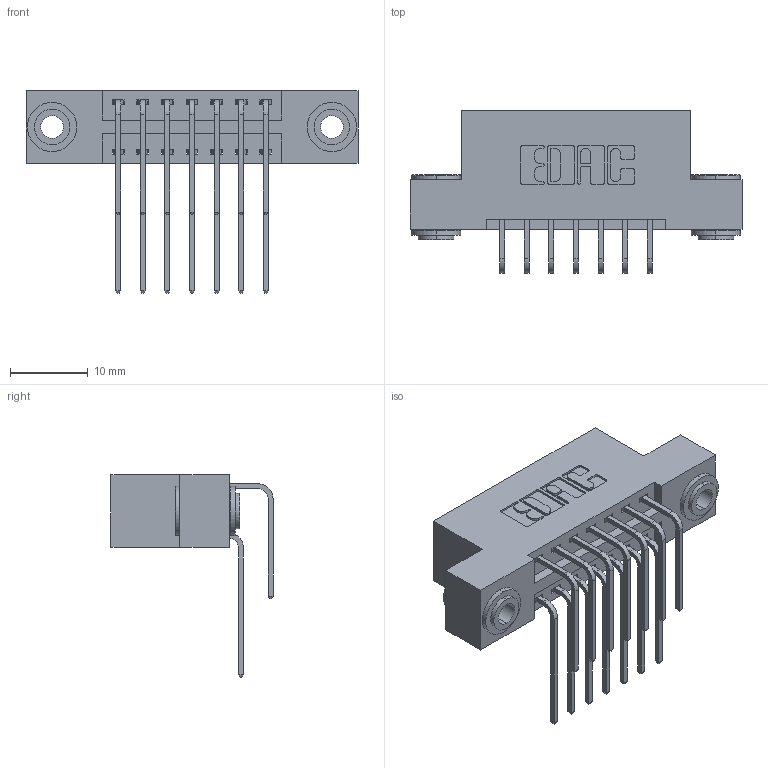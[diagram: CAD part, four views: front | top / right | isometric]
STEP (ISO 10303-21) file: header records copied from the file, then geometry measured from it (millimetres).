
FILE_DESCRIPTION (( 'STEP AP203' ), '1' );
FILE_NAME ('396-014-559-203.STEP', '2018-08-31T11:12:21', ( '' ), ( '' ), 'SwSTEP 2.0', 'SolidWorks 2016', '' );
FILE_SCHEMA (( 'CONFIG_CONTROL_DESIGN' ));
Length unit declared in the file: inch
Products named in the file (5): 346 Part_Flush Mounting Lugs - 0.156 Dia-TH; 345-292-001_558 559 Tail - 1; 345-292-001_559 Tail - 2; 345-250-002_345-250-002-102; 396-014-559-203
Assembly tree (17 placements, depth 2):
  396-014-559-203
    346 Part_Flush Mounting Lugs - 0.156 Dia-TH
    345-292-001_558 559 Tail - 1  x7
    345-292-001_559 Tail - 2  x7
    345-250-002_345-250-002-102  x2
Bounding box: 42.8 x 20.89 x 26.16 mm (x, y, z)
Volume: 4001.8 mm3; surface area: 5552.2 mm2
Topology: 17 solids, 17 shells, 916 faces, 2659 edges, 1750 vertices
Faces by surface type: plane 604, cylinder 304, cone 8
Entity records: 11714 total; most frequent: CARTESIAN_POINT 2006, ORIENTED_EDGE 1882, DIRECTION 1823, EDGE_CURVE 941, LINE 717, VECTOR 717, VERTEX_POINT 622, AXIS2_PLACEMENT_3D 553
